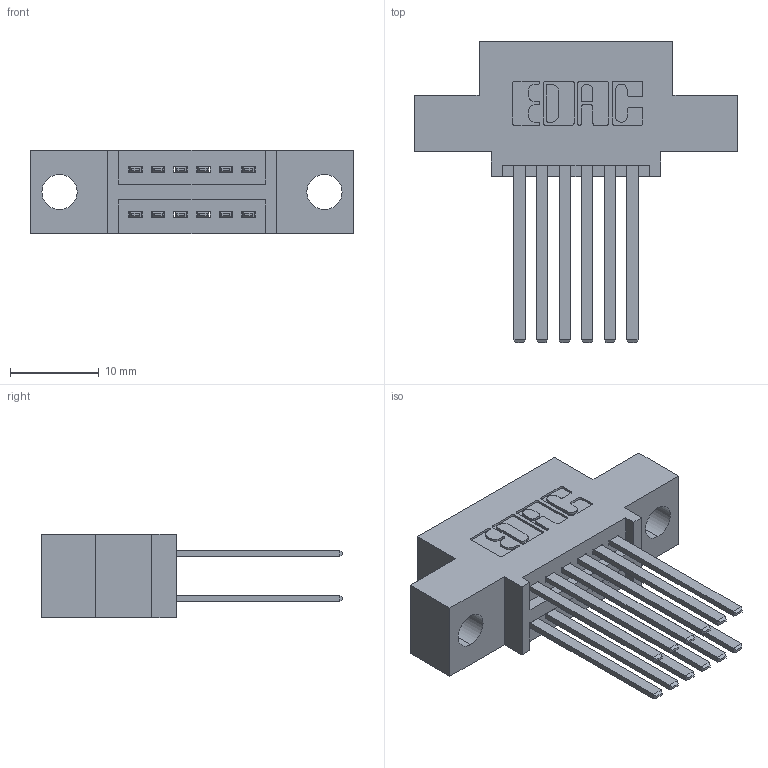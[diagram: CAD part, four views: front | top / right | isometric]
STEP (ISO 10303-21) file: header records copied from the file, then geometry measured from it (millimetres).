
FILE_DESCRIPTION (( 'STEP AP203' ), '1' );
FILE_NAME ('345-012-544-504.STEP', '2021-05-19T15:47:33', ( '' ), ( '' ), 'SwSTEP 2.0', 'SolidWorks 2020', '' );
FILE_SCHEMA (( 'CONFIG_CONTROL_DESIGN' ));
Length unit declared in the file: inch
Products named in the file (3): 345-292-001_345-293-144; 345 Part_0.110 Offset - 0.156 Dia-TI; 345-012-544-504
Assembly tree (13 placements, depth 2):
  345-012-544-504
    345 Part_0.110 Offset - 0.156 Dia-TI
    345-292-001_345-293-144  x12
Bounding box: 36.45 x 33.96 x 9.4 mm (x, y, z)
Volume: 3195.4 mm3; surface area: 4463.6 mm2
Topology: 13 solids, 13 shells, 672 faces, 1961 edges, 1290 vertices
Faces by surface type: plane 446, cylinder 226
Entity records: 9921 total; most frequent: CARTESIAN_POINT 1702, ORIENTED_EDGE 1634, DIRECTION 1541, EDGE_CURVE 817, LINE 665, VECTOR 665, VERTEX_POINT 542, AXIS2_PLACEMENT_3D 438
